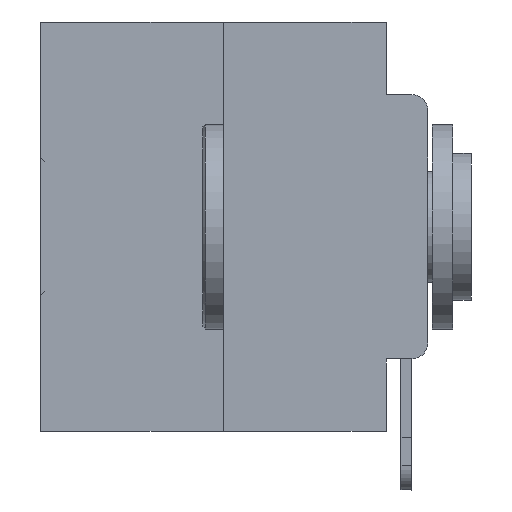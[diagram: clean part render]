
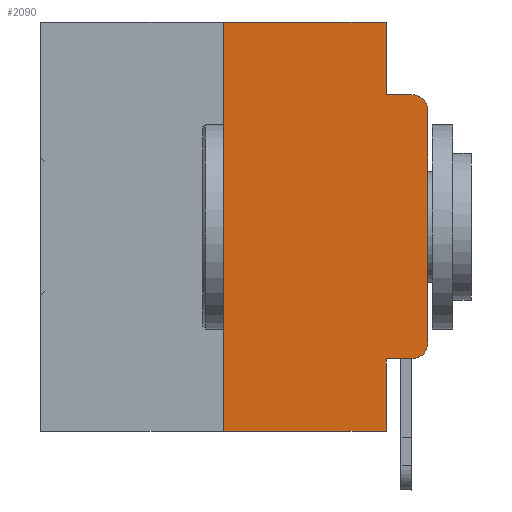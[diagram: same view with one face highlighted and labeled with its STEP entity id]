
A CAD part, left-side view. The second image highlights one B-rep face of the part: STEP entity #2090.
In plain terms, the highlighted planar face has unit normal (-1, 0, 0).
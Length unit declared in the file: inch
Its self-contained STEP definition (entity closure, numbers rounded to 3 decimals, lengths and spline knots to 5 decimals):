
#97 = DIRECTION ( 'NONE',  ( 0., 0., -1. ) ) ;
#617 = DIRECTION ( 'NONE',  ( 0., -1., 0. ) ) ;
#684 = LINE ( 'NONE', #17139, #23576 ) ;
#877 = CARTESIAN_POINT ( 'NONE',  ( 0., 0.051, 0. ) ) ;
#2090 = ADVANCED_FACE ( 'NONE', ( #22766 ), #28996, .F. ) ;
#2125 = CARTESIAN_POINT ( 'NONE',  ( 0., 0.25, -0.5 ) ) ;
#3145 = VERTEX_POINT ( 'NONE', #12812 ) ;
#4959 = VECTOR ( 'NONE', #22953, 39.37008 ) ;
#5019 = EDGE_CURVE ( 'NONE', #21269, #10281, #19678, .T. ) ;
#5694 = CARTESIAN_POINT ( 'NONE',  ( 0., 0.02, -0.0885 ) ) ;
#6631 = CARTESIAN_POINT ( 'NONE',  ( 0., 0.25, 0. ) ) ;
#7525 = EDGE_CURVE ( 'NONE', #10486, #13421, #10530, .T. ) ;
#7793 = CARTESIAN_POINT ( 'NONE',  ( 0., 0.051, 0. ) ) ;
#8204 = EDGE_CURVE ( 'NONE', #12236, #21269, #684, .T. ) ;
#8408 = VERTEX_POINT ( 'NONE', #16356 ) ;
#8539 = CARTESIAN_POINT ( 'NONE',  ( 0., 0.02, -0.1085 ) ) ;
#8551 = CARTESIAN_POINT ( 'NONE',  ( 0., 0.02, -0.3915 ) ) ;
#9080 = CARTESIAN_POINT ( 'NONE',  ( 0., 0.051, -0.0885 ) ) ;
#9285 = EDGE_CURVE ( 'NONE', #13421, #12236, #16515, .T. ) ;
#9558 = VECTOR ( 'NONE', #14895, 39.37008 ) ;
#9663 = DIRECTION ( 'NONE',  ( 0., -1., 0. ) ) ;
#9791 = DIRECTION ( 'NONE',  ( 0., 0., 1. ) ) ;
#9825 = CARTESIAN_POINT ( 'NONE',  ( 0., 0.473, 0. ) ) ;
#10281 = VERTEX_POINT ( 'NONE', #5694 ) ;
#10327 = VECTOR ( 'NONE', #617, 39.37008 ) ;
#10425 = CARTESIAN_POINT ( 'NONE',  ( 0., 0.02, -0.4115 ) ) ;
#10486 = VERTEX_POINT ( 'NONE', #2125 ) ;
#10530 = LINE ( 'NONE', #6631, #18293 ) ;
#11008 = CARTESIAN_POINT ( 'NONE',  ( 0., 0.051, -0.4115 ) ) ;
#11180 = DIRECTION ( 'NONE',  ( 0., 0., -1. ) ) ;
#12236 = VERTEX_POINT ( 'NONE', #877 ) ;
#12812 = CARTESIAN_POINT ( 'NONE',  ( 0., 0., -0.3915 ) ) ;
#13385 = ORIENTED_EDGE ( 'NONE', *, *, #29482, .T. ) ;
#13421 = VERTEX_POINT ( 'NONE', #16460 ) ;
#14280 = AXIS2_PLACEMENT_3D ( 'NONE', #8539, #26753, #11180 ) ;
#14402 = ORIENTED_EDGE ( 'NONE', *, *, #9285, .F. ) ;
#14573 = DIRECTION ( 'NONE',  ( 0., 0., 1. ) ) ;
#14895 = DIRECTION ( 'NONE',  ( 0., -1., 0. ) ) ;
#15004 = CARTESIAN_POINT ( 'NONE',  ( 0., 0.051, -0.0885 ) ) ;
#15173 = AXIS2_PLACEMENT_3D ( 'NONE', #31124, #15437, #97 ) ;
#15437 = DIRECTION ( 'NONE',  ( 1., 0., 0. ) ) ;
#16244 = DIRECTION ( 'NONE',  ( -1., 0., 0. ) ) ;
#16356 = CARTESIAN_POINT ( 'NONE',  ( 0., 0., -0.1085 ) ) ;
#16460 = CARTESIAN_POINT ( 'NONE',  ( 0., 0.25, 0. ) ) ;
#16515 = LINE ( 'NONE', #9825, #9558 ) ;
#16532 = VERTEX_POINT ( 'NONE', #16937 ) ;
#16937 = CARTESIAN_POINT ( 'NONE',  ( 0., 0.051, -0.4115 ) ) ;
#17139 = CARTESIAN_POINT ( 'NONE',  ( 0., 0.051, 0. ) ) ;
#17319 = LINE ( 'NONE', #11008, #10327 ) ;
#17743 = VECTOR ( 'NONE', #9791, 39.37008 ) ;
#17922 = EDGE_CURVE ( 'NONE', #3145, #8408, #32257, .T. ) ;
#18077 = ORIENTED_EDGE ( 'NONE', *, *, #24223, .T. ) ;
#18293 = VECTOR ( 'NONE', #14573, 39.37008 ) ;
#18988 = CIRCLE ( 'NONE', #14280, 0.02 ) ;
#19678 = LINE ( 'NONE', #15004, #4959 ) ;
#19881 = EDGE_CURVE ( 'NONE', #10486, #32260, #26481, .T. ) ;
#20490 = EDGE_LOOP ( 'NONE', ( #22845, #26123, #28575, #23329, #14402, #26153, #25450, #30982, #13385, #18077 ) ) ;
#21269 = VERTEX_POINT ( 'NONE', #9080 ) ;
#21571 = DIRECTION ( 'NONE',  ( 0., 0., -1. ) ) ;
#22766 = FACE_OUTER_BOUND ( 'NONE', #20490, .T. ) ;
#22845 = ORIENTED_EDGE ( 'NONE', *, *, #17922, .T. ) ;
#22953 = DIRECTION ( 'NONE',  ( 0., -1., 0. ) ) ;
#23329 = ORIENTED_EDGE ( 'NONE', *, *, #8204, .F. ) ;
#23576 = VECTOR ( 'NONE', #32123, 39.37008 ) ;
#24223 = EDGE_CURVE ( 'NONE', #25402, #3145, #24356, .T. ) ;
#24356 = CIRCLE ( 'NONE', #32669, 0.02 ) ;
#25402 = VERTEX_POINT ( 'NONE', #10425 ) ;
#25405 = CARTESIAN_POINT ( 'NONE',  ( 0., 0.473, -0.5 ) ) ;
#25450 = ORIENTED_EDGE ( 'NONE', *, *, #19881, .T. ) ;
#26027 = DIRECTION ( 'NONE',  ( 0., 0., -1. ) ) ;
#26123 = ORIENTED_EDGE ( 'NONE', *, *, #28682, .T. ) ;
#26153 = ORIENTED_EDGE ( 'NONE', *, *, #7525, .F. ) ;
#26481 = LINE ( 'NONE', #25405, #29288 ) ;
#26500 = CARTESIAN_POINT ( 'NONE',  ( 0., 0.051, -0.5 ) ) ;
#26753 = DIRECTION ( 'NONE',  ( -1., 0., 0. ) ) ;
#28575 = ORIENTED_EDGE ( 'NONE', *, *, #5019, .F. ) ;
#28682 = EDGE_CURVE ( 'NONE', #8408, #10281, #18988, .T. ) ;
#28996 = PLANE ( 'NONE',  #15173 ) ;
#29288 = VECTOR ( 'NONE', #9663, 39.37008 ) ;
#29482 = EDGE_CURVE ( 'NONE', #16532, #25402, #17319, .T. ) ;
#30888 = CARTESIAN_POINT ( 'NONE',  ( 0., 0., 0. ) ) ;
#30982 = ORIENTED_EDGE ( 'NONE', *, *, #32323, .F. ) ;
#31124 = CARTESIAN_POINT ( 'NONE',  ( 0., 0.473, 0. ) ) ;
#31993 = LINE ( 'NONE', #7793, #32421 ) ;
#32123 = DIRECTION ( 'NONE',  ( 0., 0., -1. ) ) ;
#32257 = LINE ( 'NONE', #30888, #17743 ) ;
#32260 = VERTEX_POINT ( 'NONE', #26500 ) ;
#32323 = EDGE_CURVE ( 'NONE', #16532, #32260, #31993, .T. ) ;
#32421 = VECTOR ( 'NONE', #26027, 39.37008 ) ;
#32669 = AXIS2_PLACEMENT_3D ( 'NONE', #8551, #16244, #21571 ) ;
